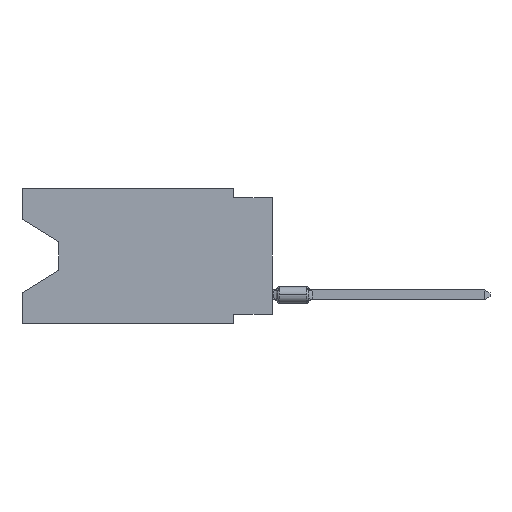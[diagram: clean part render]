
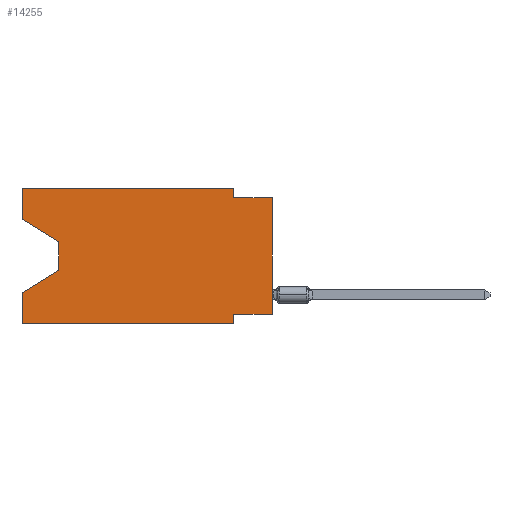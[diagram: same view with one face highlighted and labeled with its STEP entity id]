
A CAD part, left-side view. The second image highlights one B-rep face of the part: STEP entity #14255.
In plain terms, the highlighted planar face has unit normal (-1, 0, 0).
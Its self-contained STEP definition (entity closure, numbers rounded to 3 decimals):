
#23 = VERTEX_POINT ( 'NONE', #1459 ) ;
#80 = EDGE_CURVE ( 'NONE', #11281, #1887, #13380, .T. ) ;
#142 = VERTEX_POINT ( 'NONE', #7815 ) ;
#214 = VECTOR ( 'NONE', #7835, 1000. ) ;
#412 = LINE ( 'NONE', #5033, #11129 ) ;
#458 = CARTESIAN_POINT ( 'NONE',  ( 0., 0., -8.255 ) ) ;
#479 = ORIENTED_EDGE ( 'NONE', *, *, #6576, .F. ) ;
#635 = VECTOR ( 'NONE', #6427, 1000. ) ;
#751 = VERTEX_POINT ( 'NONE', #12381 ) ;
#919 = EDGE_CURVE ( 'NONE', #142, #11281, #11604, .T. ) ;
#1029 = DIRECTION ( 'NONE',  ( 0., -0.855, -0.519 ) ) ;
#1378 = AXIS2_PLACEMENT_3D ( 'NONE', #9981, #4284, #4367 ) ;
#1459 = CARTESIAN_POINT ( 'NONE',  ( 0., 0., -8.255 ) ) ;
#1462 = VERTEX_POINT ( 'NONE', #12459 ) ;
#1464 = VERTEX_POINT ( 'NONE', #6673 ) ;
#1532 = CARTESIAN_POINT ( 'NONE',  ( 0., 2.54, -8.255 ) ) ;
#1670 = EDGE_LOOP ( 'NONE', ( #7887, #3996, #8680, #479, #10411, #4285, #6649, #8930, #5975, #10402, #9193, #5296 ) ) ;
#1887 = VERTEX_POINT ( 'NONE', #5078 ) ;
#2395 = CARTESIAN_POINT ( 'NONE',  ( 0., 16.383, -6.852 ) ) ;
#2402 = CARTESIAN_POINT ( 'NONE',  ( 0., 16.383, -2.038 ) ) ;
#2553 = DIRECTION ( 'NONE',  ( 0., 0., -1. ) ) ;
#2633 = EDGE_CURVE ( 'NONE', #13842, #14386, #412, .T. ) ;
#2829 = EDGE_CURVE ( 'NONE', #23, #12853, #10330, .T. ) ;
#3097 = VECTOR ( 'NONE', #9377, 1000. ) ;
#3311 = VECTOR ( 'NONE', #5381, 1000. ) ;
#3749 = CARTESIAN_POINT ( 'NONE',  ( 0., 16.383, 0. ) ) ;
#3834 = CARTESIAN_POINT ( 'NONE',  ( 0., 0., -0.635 ) ) ;
#3996 = ORIENTED_EDGE ( 'NONE', *, *, #12762, .T. ) ;
#4284 = DIRECTION ( 'NONE',  ( 1., 0., 0. ) ) ;
#4285 = ORIENTED_EDGE ( 'NONE', *, *, #7579, .F. ) ;
#4367 = DIRECTION ( 'NONE',  ( 0., 0., -1. ) ) ;
#4421 = CARTESIAN_POINT ( 'NONE',  ( 0., 0., 0. ) ) ;
#4838 = DIRECTION ( 'NONE',  ( 0., -1., 0. ) ) ;
#5033 = CARTESIAN_POINT ( 'NONE',  ( 0., 13.97, -5.385 ) ) ;
#5078 = CARTESIAN_POINT ( 'NONE',  ( 0., 2.54, -0.635 ) ) ;
#5136 = EDGE_CURVE ( 'NONE', #1464, #1462, #11663, .T. ) ;
#5281 = VECTOR ( 'NONE', #6605, 1000. ) ;
#5296 = ORIENTED_EDGE ( 'NONE', *, *, #13866, .F. ) ;
#5381 = DIRECTION ( 'NONE',  ( 0., 0., 1. ) ) ;
#5494 = VECTOR ( 'NONE', #8381, 1000. ) ;
#5598 = CARTESIAN_POINT ( 'NONE',  ( 0., 13.97, -5.385 ) ) ;
#5734 = VECTOR ( 'NONE', #1029, 1000. ) ;
#5975 = ORIENTED_EDGE ( 'NONE', *, *, #12855, .F. ) ;
#6359 = LINE ( 'NONE', #458, #635 ) ;
#6427 = DIRECTION ( 'NONE',  ( 0., 1., 0. ) ) ;
#6576 = EDGE_CURVE ( 'NONE', #13737, #14386, #13248, .T. ) ;
#6605 = DIRECTION ( 'NONE',  ( 0., 0., -1. ) ) ;
#6649 = ORIENTED_EDGE ( 'NONE', *, *, #13668, .F. ) ;
#6673 = CARTESIAN_POINT ( 'NONE',  ( 0., 16.383, -2.038 ) ) ;
#7100 = DIRECTION ( 'NONE',  ( 0., 0., -1. ) ) ;
#7107 = LINE ( 'NONE', #8322, #9627 ) ;
#7579 = EDGE_CURVE ( 'NONE', #10446, #751, #7107, .T. ) ;
#7710 = PLANE ( 'NONE',  #1378 ) ;
#7815 = CARTESIAN_POINT ( 'NONE',  ( 0., 16.383, 0. ) ) ;
#7835 = DIRECTION ( 'NONE',  ( 0., -1., 0. ) ) ;
#7887 = ORIENTED_EDGE ( 'NONE', *, *, #5136, .T. ) ;
#7916 = EDGE_CURVE ( 'NONE', #13737, #751, #9203, .T. ) ;
#7970 = VECTOR ( 'NONE', #12861, 1000. ) ;
#8167 = LINE ( 'NONE', #11673, #10412 ) ;
#8322 = CARTESIAN_POINT ( 'NONE',  ( 0., 2.54, -8.89 ) ) ;
#8381 = DIRECTION ( 'NONE',  ( 0., 0., 1. ) ) ;
#8535 = LINE ( 'NONE', #3834, #13096 ) ;
#8680 = ORIENTED_EDGE ( 'NONE', *, *, #2633, .T. ) ;
#8930 = ORIENTED_EDGE ( 'NONE', *, *, #2829, .T. ) ;
#9193 = ORIENTED_EDGE ( 'NONE', *, *, #919, .F. ) ;
#9203 = LINE ( 'NONE', #14007, #214 ) ;
#9377 = DIRECTION ( 'NONE',  ( 0., -1., 0. ) ) ;
#9567 = DIRECTION ( 'NONE',  ( 0., 0.855, -0.519 ) ) ;
#9627 = VECTOR ( 'NONE', #2553, 1000. ) ;
#9981 = CARTESIAN_POINT ( 'NONE',  ( 0., 16.383, 0. ) ) ;
#10067 = LINE ( 'NONE', #14659, #3311 ) ;
#10091 = CARTESIAN_POINT ( 'NONE',  ( 0., 2.54, 0. ) ) ;
#10330 = LINE ( 'NONE', #4421, #7970 ) ;
#10402 = ORIENTED_EDGE ( 'NONE', *, *, #80, .F. ) ;
#10411 = ORIENTED_EDGE ( 'NONE', *, *, #7916, .T. ) ;
#10412 = VECTOR ( 'NONE', #7100, 1000. ) ;
#10446 = VERTEX_POINT ( 'NONE', #1532 ) ;
#10514 = CARTESIAN_POINT ( 'NONE',  ( 0., 16.383, 0. ) ) ;
#10737 = CARTESIAN_POINT ( 'NONE',  ( 0., 0., -0.635 ) ) ;
#11041 = FACE_OUTER_BOUND ( 'NONE', #1670, .T. ) ;
#11129 = VECTOR ( 'NONE', #9567, 1000. ) ;
#11281 = VERTEX_POINT ( 'NONE', #11758 ) ;
#11604 = LINE ( 'NONE', #10514, #3097 ) ;
#11663 = LINE ( 'NONE', #2402, #5734 ) ;
#11673 = CARTESIAN_POINT ( 'NONE',  ( 0., 13.97, -3.505 ) ) ;
#11758 = CARTESIAN_POINT ( 'NONE',  ( 0., 2.54, 0. ) ) ;
#12381 = CARTESIAN_POINT ( 'NONE',  ( 0., 2.54, -8.89 ) ) ;
#12459 = CARTESIAN_POINT ( 'NONE',  ( 0., 13.97, -3.505 ) ) ;
#12762 = EDGE_CURVE ( 'NONE', #1462, #13842, #8167, .T. ) ;
#12853 = VERTEX_POINT ( 'NONE', #10737 ) ;
#12855 = EDGE_CURVE ( 'NONE', #1887, #12853, #8535, .T. ) ;
#12861 = DIRECTION ( 'NONE',  ( 0., 0., 1. ) ) ;
#13096 = VECTOR ( 'NONE', #4838, 1000. ) ;
#13248 = LINE ( 'NONE', #3749, #5494 ) ;
#13380 = LINE ( 'NONE', #10091, #5281 ) ;
#13668 = EDGE_CURVE ( 'NONE', #23, #10446, #6359, .T. ) ;
#13737 = VERTEX_POINT ( 'NONE', #14349 ) ;
#13842 = VERTEX_POINT ( 'NONE', #5598 ) ;
#13866 = EDGE_CURVE ( 'NONE', #1464, #142, #10067, .T. ) ;
#14007 = CARTESIAN_POINT ( 'NONE',  ( 0., 16.383, -8.89 ) ) ;
#14255 = ADVANCED_FACE ( 'NONE', ( #11041 ), #7710, .F. ) ;
#14349 = CARTESIAN_POINT ( 'NONE',  ( 0., 16.383, -8.89 ) ) ;
#14386 = VERTEX_POINT ( 'NONE', #2395 ) ;
#14659 = CARTESIAN_POINT ( 'NONE',  ( 0., 16.383, 0. ) ) ;
